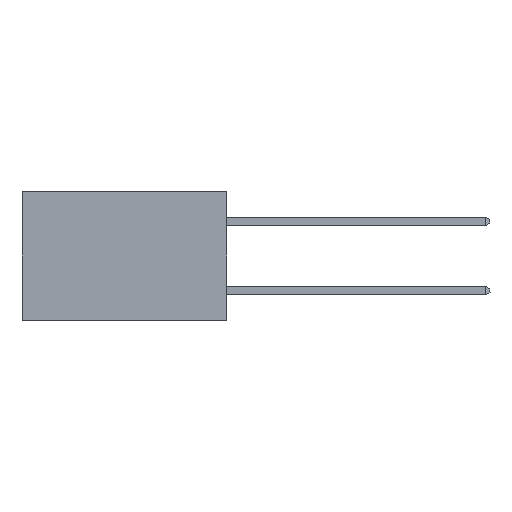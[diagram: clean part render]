
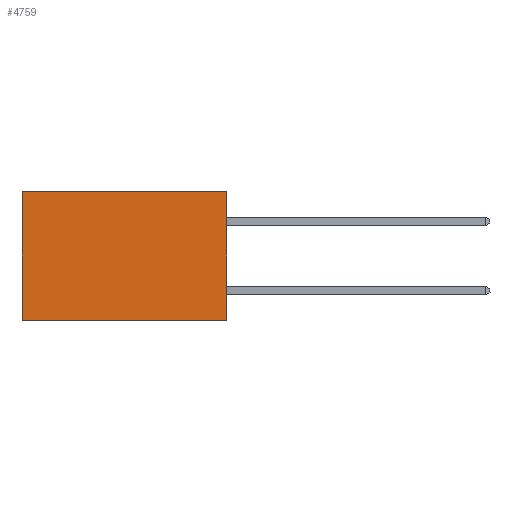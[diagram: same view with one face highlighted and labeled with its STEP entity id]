
A CAD part, left-side view. The second image highlights one B-rep face of the part: STEP entity #4759.
In plain terms, the highlighted planar face has unit normal (-1, 0, 0).
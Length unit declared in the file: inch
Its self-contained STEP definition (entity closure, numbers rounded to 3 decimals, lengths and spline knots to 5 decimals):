
#847 = VERTEX_POINT ( 'NONE', #9014 ) ;
#1212 = LINE ( 'NONE', #4878, #13020 ) ;
#1398 = DIRECTION ( 'NONE',  ( 0., 0., -1. ) ) ;
#1720 = AXIS2_PLACEMENT_3D ( 'NONE', #2505, #8263, #1398 ) ;
#2505 = CARTESIAN_POINT ( 'NONE',  ( 0.277, 0., -0.37 ) ) ;
#2654 = DIRECTION ( 'NONE',  ( 0., 0., -1. ) ) ;
#3114 = VECTOR ( 'NONE', #10276, 39.37008 ) ;
#3178 = LINE ( 'NONE', #9687, #14262 ) ;
#3442 = EDGE_CURVE ( 'NONE', #14585, #13787, #1212, .T. ) ;
#3602 = PLANE ( 'NONE',  #1720 ) ;
#3885 = CARTESIAN_POINT ( 'NONE',  ( 0.277, 0., 0. ) ) ;
#4064 = ORIENTED_EDGE ( 'NONE', *, *, #11693, .T. ) ;
#4195 = VERTEX_POINT ( 'NONE', #3885 ) ;
#4759 = ADVANCED_FACE ( 'NONE', ( #4946 ), #3602, .F. ) ;
#4878 = CARTESIAN_POINT ( 'NONE',  ( 0.277, 0.59, -0.37 ) ) ;
#4946 = FACE_OUTER_BOUND ( 'NONE', #6526, .T. ) ;
#5067 = DIRECTION ( 'NONE',  ( 0., 0., -1. ) ) ;
#5698 = CARTESIAN_POINT ( 'NONE',  ( 0.277, 0., 0. ) ) ;
#6526 = EDGE_LOOP ( 'NONE', ( #13408, #8858, #13827, #4064 ) ) ;
#7173 = CARTESIAN_POINT ( 'NONE',  ( 0.277, 0.59, -0.37 ) ) ;
#7897 = CARTESIAN_POINT ( 'NONE',  ( 0.277, 0., -0.37 ) ) ;
#8263 = DIRECTION ( 'NONE',  ( 1., 0., 0. ) ) ;
#8858 = ORIENTED_EDGE ( 'NONE', *, *, #12855, .F. ) ;
#9014 = CARTESIAN_POINT ( 'NONE',  ( 0.277, 0., -0.37 ) ) ;
#9687 = CARTESIAN_POINT ( 'NONE',  ( 0.277, 0., -0.37 ) ) ;
#9975 = EDGE_CURVE ( 'NONE', #4195, #847, #3178, .T. ) ;
#10276 = DIRECTION ( 'NONE',  ( 0., 1., 0. ) ) ;
#10804 = LINE ( 'NONE', #7897, #13466 ) ;
#11693 = EDGE_CURVE ( 'NONE', #4195, #14585, #12224, .T. ) ;
#12224 = LINE ( 'NONE', #5698, #3114 ) ;
#12855 = EDGE_CURVE ( 'NONE', #847, #13787, #10804, .T. ) ;
#13020 = VECTOR ( 'NONE', #2654, 39.37008 ) ;
#13408 = ORIENTED_EDGE ( 'NONE', *, *, #3442, .T. ) ;
#13466 = VECTOR ( 'NONE', #13572, 39.37008 ) ;
#13572 = DIRECTION ( 'NONE',  ( 0., 1., 0. ) ) ;
#13787 = VERTEX_POINT ( 'NONE', #7173 ) ;
#13827 = ORIENTED_EDGE ( 'NONE', *, *, #9975, .F. ) ;
#14262 = VECTOR ( 'NONE', #5067, 39.37008 ) ;
#14329 = CARTESIAN_POINT ( 'NONE',  ( 0.277, 0.59, 0. ) ) ;
#14585 = VERTEX_POINT ( 'NONE', #14329 ) ;
